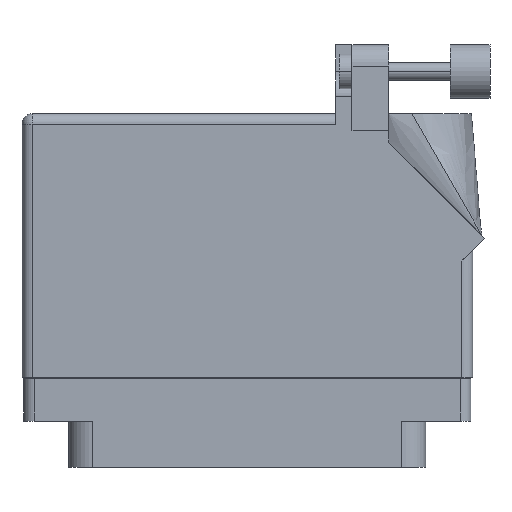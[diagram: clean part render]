
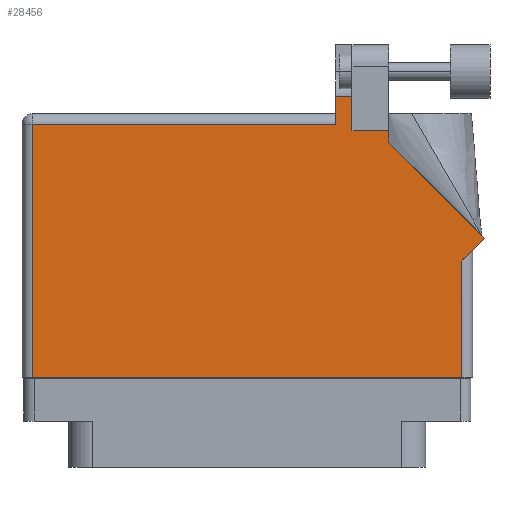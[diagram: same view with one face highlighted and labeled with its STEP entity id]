
A CAD part, front view. The second image highlights one B-rep face of the part: STEP entity #28456.
In plain terms, the highlighted face is planar.
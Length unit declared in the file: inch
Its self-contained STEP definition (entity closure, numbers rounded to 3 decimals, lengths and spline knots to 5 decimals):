
#218 = CARTESIAN_POINT ( 'NONE',  ( 0.607, 1.33, 0.455 ) ) ;
#1058 = ORIENTED_EDGE ( 'NONE', *, *, #24238, .T. ) ;
#1431 = EDGE_CURVE ( 'NONE', #20812, #7637, #4890, .T. ) ;
#1610 = VECTOR ( 'NONE', #19747, 39.37008 ) ;
#2135 = CARTESIAN_POINT ( 'NONE',  ( 0.513, 1.368, 0.455 ) ) ;
#3931 = AXIS2_PLACEMENT_3D ( 'NONE', #35002, #35348, #38730 ) ;
#4875 = VECTOR ( 'NONE', #38508, 39.37008 ) ;
#4890 = LINE ( 'NONE', #34537, #26949 ) ;
#5059 = LINE ( 'NONE', #46014, #36031 ) ;
#5750 = VERTEX_POINT ( 'NONE', #2135 ) ;
#6228 = DIRECTION ( 'NONE',  ( 0.707, 0.707, 0. ) ) ;
#6939 = VECTOR ( 'NONE', #43112, 39.37008 ) ;
#7637 = VERTEX_POINT ( 'NONE', #51343 ) ;
#7805 = CARTESIAN_POINT ( 'NONE',  ( 0.82, 1.33, 0.455 ) ) ;
#8727 = EDGE_CURVE ( 'NONE', #48734, #19745, #38965, .T. ) ;
#8790 = VERTEX_POINT ( 'NONE', #23964 ) ;
#11113 = LINE ( 'NONE', #32164, #41451 ) ;
#12524 = ORIENTED_EDGE ( 'NONE', *, *, #29941, .T. ) ;
#12625 = ORIENTED_EDGE ( 'NONE', *, *, #8727, .T. ) ;
#12676 = LINE ( 'NONE', #30718, #6939 ) ;
#13054 = VECTOR ( 'NONE', #6228, 39.37008 ) ;
#13086 = VERTEX_POINT ( 'NONE', #18698 ) ;
#13358 = DIRECTION ( 'NONE',  ( 0., 1., 0. ) ) ;
#13407 = EDGE_CURVE ( 'NONE', #8790, #5750, #39508, .T. ) ;
#15036 = CARTESIAN_POINT ( 'NONE',  ( 1.37671, 0.70771, 0.455 ) ) ;
#16965 = VERTEX_POINT ( 'NONE', #7805 ) ;
#17886 = PLANE ( 'NONE',  #3931 ) ;
#18465 = DIRECTION ( 'NONE',  ( 0., 1., 0. ) ) ;
#18543 = CARTESIAN_POINT ( 'NONE',  ( -1.306, -0.1, 0.455 ) ) ;
#18698 = CARTESIAN_POINT ( 'NONE',  ( -1.244, 1.368, 0.455 ) ) ;
#18966 = VECTOR ( 'NONE', #13358, 39.37008 ) ;
#19745 = VERTEX_POINT ( 'NONE', #40899 ) ;
#19747 = DIRECTION ( 'NONE',  ( 0., -1., 0. ) ) ;
#20016 = VECTOR ( 'NONE', #39550, 39.37008 ) ;
#20258 = VECTOR ( 'NONE', #39924, 39.37008 ) ;
#20517 = VECTOR ( 'NONE', #28796, 39.37008 ) ;
#20812 = VERTEX_POINT ( 'NONE', #218 ) ;
#20900 = EDGE_CURVE ( 'NONE', #5750, #13086, #11113, .T. ) ;
#21288 = CARTESIAN_POINT ( 'NONE',  ( 1.244, 0.575, 0.455 ) ) ;
#21775 = LINE ( 'NONE', #28962, #20517 ) ;
#21837 = DIRECTION ( 'NONE',  ( -1., 0., 0. ) ) ;
#23964 = CARTESIAN_POINT ( 'NONE',  ( 0.513, 1.5315, 0.455 ) ) ;
#24066 = LINE ( 'NONE', #38419, #20258 ) ;
#24238 = EDGE_CURVE ( 'NONE', #7637, #8790, #5059, .T. ) ;
#26014 = EDGE_CURVE ( 'NONE', #13086, #51588, #24066, .T. ) ;
#26645 = CARTESIAN_POINT ( 'NONE',  ( 1.244, -0.1, 0.455 ) ) ;
#26949 = VECTOR ( 'NONE', #18465, 39.37008 ) ;
#28456 = ADVANCED_FACE ( 'NONE', ( #51560 ), #17886, .F. ) ;
#28796 = DIRECTION ( 'NONE',  ( -1., 0., 0. ) ) ;
#28962 = CARTESIAN_POINT ( 'NONE',  ( 0.82, 1.33, 0.455 ) ) ;
#29808 = ORIENTED_EDGE ( 'NONE', *, *, #47312, .T. ) ;
#29941 = EDGE_CURVE ( 'NONE', #36269, #48734, #45825, .T. ) ;
#30718 = CARTESIAN_POINT ( 'NONE',  ( 1.244, 0.637, 0.455 ) ) ;
#31584 = EDGE_LOOP ( 'NONE', ( #42906, #1058, #39187, #45750, #41764, #29808, #36144, #12524, #12625, #50118, #39384 ) ) ;
#31712 = CARTESIAN_POINT ( 'NONE',  ( 1.37671, 0.70771, 0.455 ) ) ;
#32164 = CARTESIAN_POINT ( 'NONE',  ( -1.306, 1.368, 0.455 ) ) ;
#34537 = CARTESIAN_POINT ( 'NONE',  ( 0.607, 1.33, 0.455 ) ) ;
#35002 = CARTESIAN_POINT ( 'NONE',  ( -1.306, 1.43, 0.455 ) ) ;
#35348 = DIRECTION ( 'NONE',  ( 0., 0., -1. ) ) ;
#35814 = CARTESIAN_POINT ( 'NONE',  ( 0.513, 1.43, 0.455 ) ) ;
#36031 = VECTOR ( 'NONE', #21837, 39.37008 ) ;
#36144 = ORIENTED_EDGE ( 'NONE', *, *, #45915, .T. ) ;
#36237 = DIRECTION ( 'NONE',  ( -1., 0., 0. ) ) ;
#36269 = VERTEX_POINT ( 'NONE', #21288 ) ;
#38419 = CARTESIAN_POINT ( 'NONE',  ( -1.244, -0.1, 0.455 ) ) ;
#38508 = DIRECTION ( 'NONE',  ( 1., 0., 0. ) ) ;
#38730 = DIRECTION ( 'NONE',  ( -1., 0., 0. ) ) ;
#38965 = LINE ( 'NONE', #15036, #20016 ) ;
#39187 = ORIENTED_EDGE ( 'NONE', *, *, #13407, .T. ) ;
#39384 = ORIENTED_EDGE ( 'NONE', *, *, #44561, .T. ) ;
#39508 = LINE ( 'NONE', #35814, #1610 ) ;
#39550 = DIRECTION ( 'NONE',  ( -0.707, 0.707, 0. ) ) ;
#39924 = DIRECTION ( 'NONE',  ( 0., -1., 0. ) ) ;
#40899 = CARTESIAN_POINT ( 'NONE',  ( 0.82, 1.26442, 0.455 ) ) ;
#41451 = VECTOR ( 'NONE', #36237, 39.37008 ) ;
#41764 = ORIENTED_EDGE ( 'NONE', *, *, #26014, .T. ) ;
#42334 = LINE ( 'NONE', #46152, #18966 ) ;
#42906 = ORIENTED_EDGE ( 'NONE', *, *, #1431, .T. ) ;
#43112 = DIRECTION ( 'NONE',  ( 0., 1., 0. ) ) ;
#44561 = EDGE_CURVE ( 'NONE', #16965, #20812, #21775, .T. ) ;
#45750 = ORIENTED_EDGE ( 'NONE', *, *, #20900, .T. ) ;
#45825 = LINE ( 'NONE', #46490, #13054 ) ;
#45915 = EDGE_CURVE ( 'NONE', #50749, #36269, #12676, .T. ) ;
#46014 = CARTESIAN_POINT ( 'NONE',  ( 0.93777, 1.5315, 0.455 ) ) ;
#46017 = CARTESIAN_POINT ( 'NONE',  ( -1.244, -0.1, 0.455 ) ) ;
#46152 = CARTESIAN_POINT ( 'NONE',  ( 0.82, 1.26442, 0.455 ) ) ;
#46490 = CARTESIAN_POINT ( 'NONE',  ( 1.306, 0.637, 0.455 ) ) ;
#47312 = EDGE_CURVE ( 'NONE', #51588, #50749, #47810, .T. ) ;
#47810 = LINE ( 'NONE', #18543, #4875 ) ;
#48734 = VERTEX_POINT ( 'NONE', #31712 ) ;
#50118 = ORIENTED_EDGE ( 'NONE', *, *, #52119, .T. ) ;
#50749 = VERTEX_POINT ( 'NONE', #26645 ) ;
#51343 = CARTESIAN_POINT ( 'NONE',  ( 0.607, 1.5315, 0.455 ) ) ;
#51560 = FACE_OUTER_BOUND ( 'NONE', #31584, .T. ) ;
#51588 = VERTEX_POINT ( 'NONE', #46017 ) ;
#52119 = EDGE_CURVE ( 'NONE', #19745, #16965, #42334, .T. ) ;
